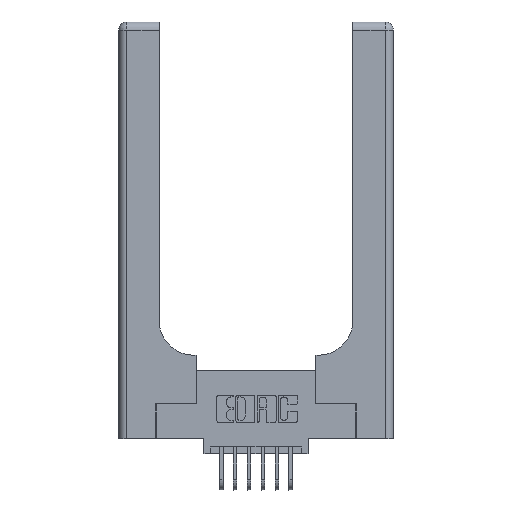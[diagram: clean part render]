
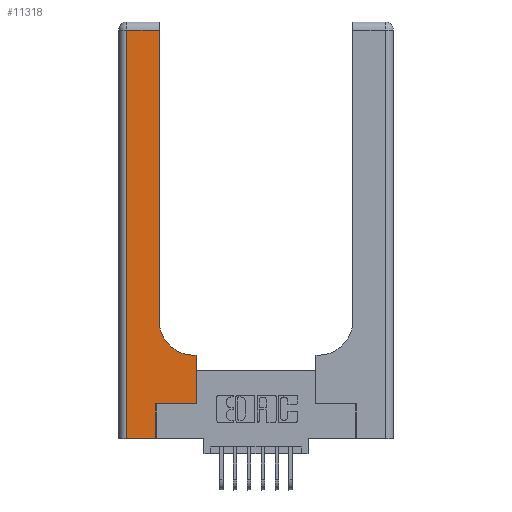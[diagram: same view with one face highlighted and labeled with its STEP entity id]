
A CAD part, top view. The second image highlights one B-rep face of the part: STEP entity #11318.
In plain terms, the highlighted planar face has unit normal (0, 0, 1).
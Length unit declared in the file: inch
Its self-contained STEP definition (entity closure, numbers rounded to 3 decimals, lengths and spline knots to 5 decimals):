
#26 = CARTESIAN_POINT ( 'NONE',  ( 0.269, 0., 0.37 ) ) ;
#92 = CARTESIAN_POINT ( 'NONE',  ( 0.5585, 0.25, 0.37 ) ) ;
#280 = CARTESIAN_POINT ( 'NONE',  ( 0.2915, 0.6, 0.37 ) ) ;
#371 = VECTOR ( 'NONE', #1315, 39.37008 ) ;
#512 = ORIENTED_EDGE ( 'NONE', *, *, #3807, .T. ) ;
#796 = VECTOR ( 'NONE', #4183, 39.37008 ) ;
#1092 = DIRECTION ( 'NONE',  ( 0., -1., 0. ) ) ;
#1315 = DIRECTION ( 'NONE',  ( 0., 1., 0. ) ) ;
#1489 = FACE_OUTER_BOUND ( 'NONE', #14693, .T. ) ;
#2309 = CARTESIAN_POINT ( 'NONE',  ( 0., 0., 0.37 ) ) ;
#2370 = LINE ( 'NONE', #12466, #15940 ) ;
#2511 = AXIS2_PLACEMENT_3D ( 'NONE', #4317, #4095, #9212 ) ;
#3160 = VERTEX_POINT ( 'NONE', #15810 ) ;
#3322 = LINE ( 'NONE', #7495, #6698 ) ;
#3620 = LINE ( 'NONE', #2309, #5236 ) ;
#3745 = CARTESIAN_POINT ( 'NONE',  ( 0.2915, 2.94, 0.37 ) ) ;
#3807 = EDGE_CURVE ( 'NONE', #10050, #6678, #10213, .T. ) ;
#4095 = DIRECTION ( 'NONE',  ( 0., 0., -1. ) ) ;
#4098 = LINE ( 'NONE', #8062, #9677 ) ;
#4183 = DIRECTION ( 'NONE',  ( -1., 0., 0. ) ) ;
#4277 = LINE ( 'NONE', #5953, #12458 ) ;
#4283 = CARTESIAN_POINT ( 'NONE',  ( 0.2915, 0.85, 0.37 ) ) ;
#4317 = CARTESIAN_POINT ( 'NONE',  ( 0., 3., 0.37 ) ) ;
#4399 = DIRECTION ( 'NONE',  ( 1., 0., 0. ) ) ;
#4589 = CARTESIAN_POINT ( 'NONE',  ( 0.5585, 0.25, 0.37 ) ) ;
#4667 = EDGE_CURVE ( 'NONE', #6131, #10906, #13979, .T. ) ;
#5088 = CARTESIAN_POINT ( 'NONE',  ( 0.269, 0.25, 0.37 ) ) ;
#5184 = EDGE_CURVE ( 'NONE', #12572, #6131, #9153, .T. ) ;
#5222 = VECTOR ( 'NONE', #4399, 39.37008 ) ;
#5236 = VECTOR ( 'NONE', #10217, 39.37008 ) ;
#5483 = ORIENTED_EDGE ( 'NONE', *, *, #6273, .T. ) ;
#5891 = EDGE_CURVE ( 'NONE', #6678, #12572, #14363, .T. ) ;
#5953 = CARTESIAN_POINT ( 'NONE',  ( 0.269, 0., 0.37 ) ) ;
#6131 = VERTEX_POINT ( 'NONE', #6992 ) ;
#6273 = EDGE_CURVE ( 'NONE', #8196, #14912, #2370, .T. ) ;
#6678 = VERTEX_POINT ( 'NONE', #4589 ) ;
#6698 = VECTOR ( 'NONE', #1092, 39.37008 ) ;
#6992 = CARTESIAN_POINT ( 'NONE',  ( 0.5415, 0.6, 0.37 ) ) ;
#7050 = CARTESIAN_POINT ( 'NONE',  ( 0.5585, 0.6, 0.37 ) ) ;
#7198 = EDGE_CURVE ( 'NONE', #3160, #11207, #3620, .T. ) ;
#7475 = ORIENTED_EDGE ( 'NONE', *, *, #5184, .T. ) ;
#7495 = CARTESIAN_POINT ( 'NONE',  ( 0.06, 3., 0.37 ) ) ;
#7955 = ORIENTED_EDGE ( 'NONE', *, *, #13975, .T. ) ;
#8062 = CARTESIAN_POINT ( 'NONE',  ( 0.2915, 3., 0.37 ) ) ;
#8196 = VERTEX_POINT ( 'NONE', #3745 ) ;
#8207 = CARTESIAN_POINT ( 'NONE',  ( 0.5415, 0.85, 0.37 ) ) ;
#8394 = DIRECTION ( 'NONE',  ( 0., 1., 0. ) ) ;
#9153 = LINE ( 'NONE', #280, #796 ) ;
#9212 = DIRECTION ( 'NONE',  ( -1., 0., 0. ) ) ;
#9316 = PLANE ( 'NONE',  #2511 ) ;
#9367 = DIRECTION ( 'NONE',  ( 1., 0., 0. ) ) ;
#9677 = VECTOR ( 'NONE', #13186, 39.37008 ) ;
#9854 = ORIENTED_EDGE ( 'NONE', *, *, #7198, .T. ) ;
#10050 = VERTEX_POINT ( 'NONE', #5088 ) ;
#10158 = CARTESIAN_POINT ( 'NONE',  ( 0.06, 2.94, 0.37 ) ) ;
#10213 = LINE ( 'NONE', #16419, #5222 ) ;
#10217 = DIRECTION ( 'NONE',  ( 1., 0., 0. ) ) ;
#10776 = ORIENTED_EDGE ( 'NONE', *, *, #4667, .T. ) ;
#10906 = VERTEX_POINT ( 'NONE', #4283 ) ;
#11136 = EDGE_CURVE ( 'NONE', #14912, #3160, #3322, .T. ) ;
#11207 = VERTEX_POINT ( 'NONE', #26 ) ;
#11287 = AXIS2_PLACEMENT_3D ( 'NONE', #8207, #11838, #9367 ) ;
#11318 = ADVANCED_FACE ( 'NONE', ( #1489 ), #9316, .F. ) ;
#11838 = DIRECTION ( 'NONE',  ( 0., 0., -1. ) ) ;
#12458 = VECTOR ( 'NONE', #8394, 39.37008 ) ;
#12466 = CARTESIAN_POINT ( 'NONE',  ( 0., 2.94, 0.37 ) ) ;
#12572 = VERTEX_POINT ( 'NONE', #7050 ) ;
#12680 = ORIENTED_EDGE ( 'NONE', *, *, #15647, .T. ) ;
#13186 = DIRECTION ( 'NONE',  ( 0., 1., 0. ) ) ;
#13586 = DIRECTION ( 'NONE',  ( -1., 0., 0. ) ) ;
#13975 = EDGE_CURVE ( 'NONE', #11207, #10050, #4277, .T. ) ;
#13979 = CIRCLE ( 'NONE', #11287, 0.25 ) ;
#14359 = ORIENTED_EDGE ( 'NONE', *, *, #5891, .T. ) ;
#14363 = LINE ( 'NONE', #92, #371 ) ;
#14586 = ORIENTED_EDGE ( 'NONE', *, *, #11136, .T. ) ;
#14693 = EDGE_LOOP ( 'NONE', ( #12680, #5483, #14586, #9854, #7955, #512, #14359, #7475, #10776 ) ) ;
#14912 = VERTEX_POINT ( 'NONE', #10158 ) ;
#15647 = EDGE_CURVE ( 'NONE', #10906, #8196, #4098, .T. ) ;
#15810 = CARTESIAN_POINT ( 'NONE',  ( 0.06, 0., 0.37 ) ) ;
#15940 = VECTOR ( 'NONE', #13586, 39.37008 ) ;
#16419 = CARTESIAN_POINT ( 'NONE',  ( 0.269, 0.25, 0.37 ) ) ;
